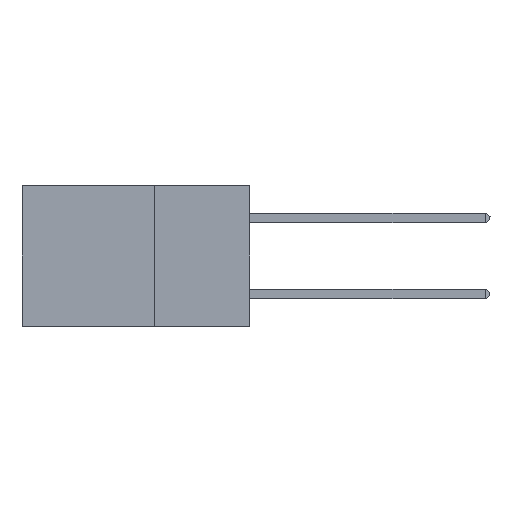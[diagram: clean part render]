
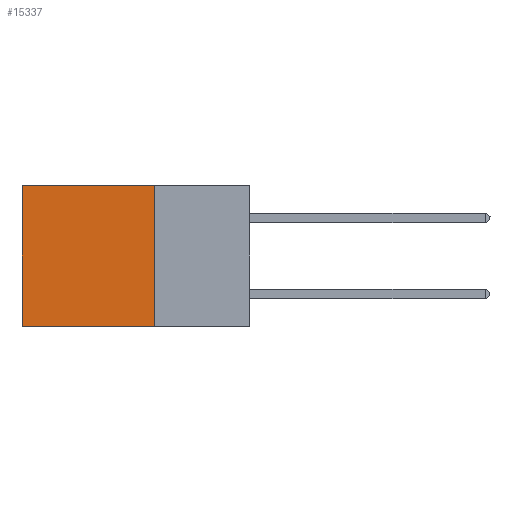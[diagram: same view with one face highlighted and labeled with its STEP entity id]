
A CAD part, left-side view. The second image highlights one B-rep face of the part: STEP entity #15337.
In plain terms, the highlighted planar face has unit normal (-1, 0, 0).
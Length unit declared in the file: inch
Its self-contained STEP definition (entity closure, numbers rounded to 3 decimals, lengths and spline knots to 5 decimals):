
#2180 = CARTESIAN_POINT ( 'NONE',  ( 0.2875, 0.6, 0. ) ) ;
#6466 = DIRECTION ( 'NONE',  ( 0., 1., 0. ) ) ;
#6678 = CARTESIAN_POINT ( 'NONE',  ( 0.2875, 0.25, 0. ) ) ;
#6963 = LINE ( 'NONE', #19251, #35840 ) ;
#7132 = VECTOR ( 'NONE', #6466, 39.37008 ) ;
#7337 = DIRECTION ( 'NONE',  ( 0., 0., -1. ) ) ;
#7566 = EDGE_CURVE ( 'NONE', #13231, #25330, #16125, .T. ) ;
#9518 = VECTOR ( 'NONE', #25283, 39.37008 ) ;
#10721 = LINE ( 'NONE', #27044, #31597 ) ;
#11114 = CARTESIAN_POINT ( 'NONE',  ( 0.2875, 0.6, -0.37 ) ) ;
#11345 = ORIENTED_EDGE ( 'NONE', *, *, #34463, .T. ) ;
#13231 = VERTEX_POINT ( 'NONE', #15847 ) ;
#14566 = VERTEX_POINT ( 'NONE', #2180 ) ;
#14951 = AXIS2_PLACEMENT_3D ( 'NONE', #30019, #35258, #24892 ) ;
#15337 = ADVANCED_FACE ( 'NONE', ( #37424 ), #21302, .F. ) ;
#15847 = CARTESIAN_POINT ( 'NONE',  ( 0.2875, 0.25, -0.37 ) ) ;
#16125 = LINE ( 'NONE', #29064, #9518 ) ;
#16268 = DIRECTION ( 'NONE',  ( 0., 0., -1. ) ) ;
#19251 = CARTESIAN_POINT ( 'NONE',  ( 0.2875, 0.25, 0. ) ) ;
#21302 = PLANE ( 'NONE',  #14951 ) ;
#22300 = ORIENTED_EDGE ( 'NONE', *, *, #31103, .T. ) ;
#22771 = LINE ( 'NONE', #26164, #7132 ) ;
#24005 = EDGE_LOOP ( 'NONE', ( #11345, #37127, #32672, #22300 ) ) ;
#24892 = DIRECTION ( 'NONE',  ( 0., 0., -1. ) ) ;
#25283 = DIRECTION ( 'NONE',  ( 0., 1., 0. ) ) ;
#25330 = VERTEX_POINT ( 'NONE', #11114 ) ;
#26164 = CARTESIAN_POINT ( 'NONE',  ( 0.2875, 0.25, 0. ) ) ;
#27044 = CARTESIAN_POINT ( 'NONE',  ( 0.2875, 0.6, 0. ) ) ;
#27185 = VERTEX_POINT ( 'NONE', #6678 ) ;
#29064 = CARTESIAN_POINT ( 'NONE',  ( 0.2875, 0.25, -0.37 ) ) ;
#30019 = CARTESIAN_POINT ( 'NONE',  ( 0.2875, 0.25, 0. ) ) ;
#31103 = EDGE_CURVE ( 'NONE', #27185, #14566, #22771, .T. ) ;
#31597 = VECTOR ( 'NONE', #7337, 39.37008 ) ;
#32672 = ORIENTED_EDGE ( 'NONE', *, *, #39809, .F. ) ;
#34463 = EDGE_CURVE ( 'NONE', #14566, #25330, #10721, .T. ) ;
#35258 = DIRECTION ( 'NONE',  ( 1., 0., 0. ) ) ;
#35840 = VECTOR ( 'NONE', #16268, 39.37008 ) ;
#37127 = ORIENTED_EDGE ( 'NONE', *, *, #7566, .F. ) ;
#37424 = FACE_OUTER_BOUND ( 'NONE', #24005, .T. ) ;
#39809 = EDGE_CURVE ( 'NONE', #27185, #13231, #6963, .T. ) ;
